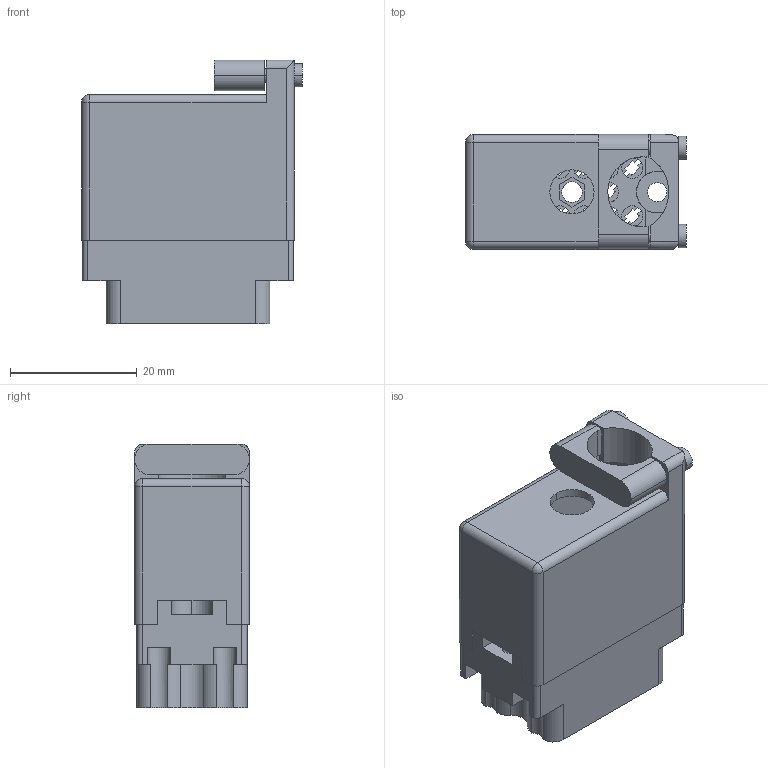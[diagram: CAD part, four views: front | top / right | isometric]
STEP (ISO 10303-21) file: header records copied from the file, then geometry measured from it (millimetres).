
FILE_DESCRIPTION (( 'STEP AP203' ), '1' );
FILE_NAME ('519-014-000-360.STEP', '2020-03-02T19:50:06', ( '' ), ( '' ), 'SwSTEP 2.0', 'SolidWorks 2016', '' );
FILE_SCHEMA (( 'CONFIG_CONTROL_DESIGN' ));
Length unit declared in the file: inch
Products named in the file (3): 519-014-000-360; 516-230-001_Metal - 020 Top Entry; 519 Plug Insulator_014
Assembly tree (2 placements, depth 2):
  519-014-000-360
    519 Plug Insulator_014
    516-230-001_Metal - 020 Top Entry
Bounding box: 34.92 x 18.16 x 41.71 mm (x, y, z)
Volume: 8807.1 mm3; surface area: 12123.6 mm2
Topology: 2 solids, 2 shells, 559 faces, 1624 edges, 1076 vertices
Faces by surface type: plane 362, cylinder 193, cone 2, sphere 2
Entity records: 18901 total; most frequent: CARTESIAN_POINT 3300, ORIENTED_EDGE 3244, DIRECTION 3198, EDGE_CURVE 1622, LINE 1162, VECTOR 1162, VERTEX_POINT 1076, AXIS2_PLACEMENT_3D 1018
